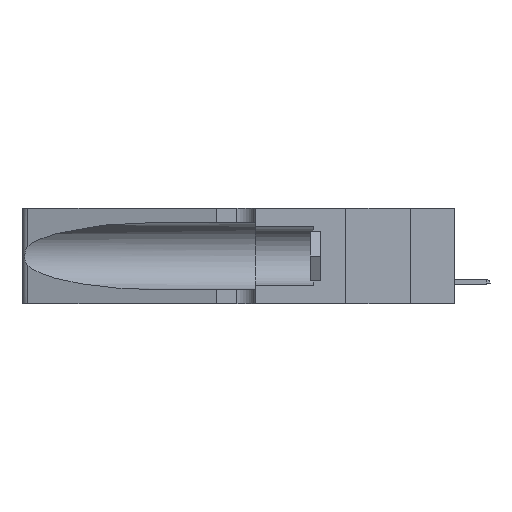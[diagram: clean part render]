
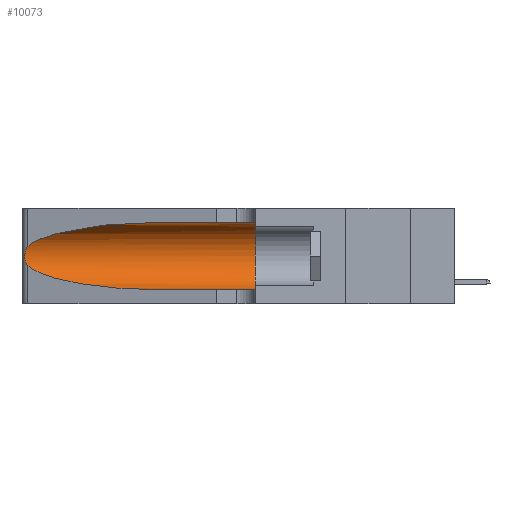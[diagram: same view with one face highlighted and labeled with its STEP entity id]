
A CAD part, left-side view. The second image highlights one B-rep face of the part: STEP entity #10073.
In plain terms, the highlighted cylindrical face has radius 3.308 mm (diameter 6.617 mm), a partial arc.
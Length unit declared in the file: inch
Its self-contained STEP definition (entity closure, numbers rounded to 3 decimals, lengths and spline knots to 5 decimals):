
#525 = DIRECTION ( 'NONE',  ( 0., -1., 0. ) ) ;
#949 = DIRECTION ( 'NONE',  ( 0., 0., -1. ) ) ;
#981 = CARTESIAN_POINT ( 'NONE',  ( 0.26075, 1.23896, 0.178 ) ) ;
#2021 = CARTESIAN_POINT ( 'NONE',  ( 0.18966, 0.96281, 0.31525 ) ) ;
#2221 = AXIS2_PLACEMENT_3D ( 'NONE', #19820, #525, #949 ) ;
#2693 = EDGE_CURVE ( 'NONE', #4115, #14118, #26232, .T. ) ;
#2950 = CARTESIAN_POINT ( 'NONE',  ( 0.25639, 1.23184, 0.21858 ) ) ;
#4115 = VERTEX_POINT ( 'NONE', #12184 ) ;
#4227 = EDGE_CURVE ( 'NONE', #4115, #12556, #16961, .T. ) ;
#4262 = CARTESIAN_POINT ( 'NONE',  ( 0.25487, 1.22718, 0.22369 ) ) ;
#4934 = CARTESIAN_POINT ( 'NONE',  ( 0.25555, 1.22993, 0.14849 ) ) ;
#5211 = CARTESIAN_POINT ( 'NONE',  ( 0.26017, 1.23833, 0.17102 ) ) ;
#5354 = CARTESIAN_POINT ( 'NONE',  ( 0.26075, 1.23896, 0.19203 ) ) ;
#6523 = CARTESIAN_POINT ( 'NONE',  ( 0.2373, 1.15595, 0.28018 ) ) ;
#6920 = CARTESIAN_POINT ( 'NONE',  ( 0.1305, 0.35, 0.05475 ) ) ;
#7315 = ORIENTED_EDGE ( 'NONE', *, *, #9658, .T. ) ;
#8468 = CARTESIAN_POINT ( 'NONE',  ( 0.2373, 1.15595, 0.08982 ) ) ;
#8658 = CARTESIAN_POINT ( 'NONE',  ( 0.1305, 0.72297, 0.31525 ) ) ;
#8821 = DIRECTION ( 'NONE',  ( 0., 0., 1. ) ) ;
#9414 = VERTEX_POINT ( 'NONE', #6920 ) ;
#9658 = EDGE_CURVE ( 'NONE', #12556, #23799, #11583, .T. ) ;
#9897 = CARTESIAN_POINT ( 'NONE',  ( 0.25487, 1.22718, 0.14631 ) ) ;
#10017 = CARTESIAN_POINT ( 'NONE',  ( 0.1305, 0.72297, 0.05475 ) ) ;
#10073 = ADVANCED_FACE ( 'NONE', ( #15599 ), #11262, .F. ) ;
#10475 =( BOUNDED_CURVE ( )  B_SPLINE_CURVE ( 3, ( #16762, #8468, #23089, #10017 ),
 .UNSPECIFIED., .F., .F. ) 
 B_SPLINE_CURVE_WITH_KNOTS ( ( 4, 4 ),
 ( 3.44316, 4.71239 ),
 .UNSPECIFIED. ) 
 CURVE ( )  GEOMETRIC_REPRESENTATION_ITEM ( )  RATIONAL_B_SPLINE_CURVE ( ( 1., 0.87, 0.87, 1. ) ) 
 REPRESENTATION_ITEM ( '' )  );
#10913 = EDGE_CURVE ( 'NONE', #23799, #18784, #10475, .T. ) ;
#11002 = LINE ( 'NONE', #19565, #17062 ) ;
#11262 = CYLINDRICAL_SURFACE ( 'NONE', #2221, 0.13025 ) ;
#11569 = CARTESIAN_POINT ( 'NONE',  ( 0.25487, 1.22718, 0.14631 ) ) ;
#11583 = B_SPLINE_CURVE_WITH_KNOTS ( 'NONE', 3,
 ( #22658, #16201, #2950, #24489, #17755, #15634, #5354, #981, #5211, #13813, #26738, #24213, #4934, #11569 ),
 .UNSPECIFIED., .F., .F.,
 ( 4, 2, 2, 2, 2, 2, 4 ),
 ( 0., 0.00027, 0.00053, 0.00107, 0.0016, 0.00187, 0.00214 ),
 .UNSPECIFIED. ) ;
#11917 = EDGE_CURVE ( 'NONE', #14118, #9414, #12728, .T. ) ;
#12184 = CARTESIAN_POINT ( 'NONE',  ( 0.1305, 0.72297, 0.31525 ) ) ;
#12556 = VERTEX_POINT ( 'NONE', #26222 ) ;
#12728 = CIRCLE ( 'NONE', #26154, 0.13025 ) ;
#13235 = EDGE_LOOP ( 'NONE', ( #14800, #7315, #13441, #21257, #23522, #22149 ) ) ;
#13441 = ORIENTED_EDGE ( 'NONE', *, *, #10913, .T. ) ;
#13813 = CARTESIAN_POINT ( 'NONE',  ( 0.25856, 1.23593, 0.16098 ) ) ;
#14118 = VERTEX_POINT ( 'NONE', #16528 ) ;
#14718 = DIRECTION ( 'NONE',  ( 0., 1., 0. ) ) ;
#14800 = ORIENTED_EDGE ( 'NONE', *, *, #4227, .T. ) ;
#15599 = FACE_OUTER_BOUND ( 'NONE', #13235, .T. ) ;
#15634 = CARTESIAN_POINT ( 'NONE',  ( 0.26018, 1.23835, 0.19895 ) ) ;
#16201 = CARTESIAN_POINT ( 'NONE',  ( 0.25555, 1.22994, 0.2215 ) ) ;
#16528 = CARTESIAN_POINT ( 'NONE',  ( 0.1305, 0.35, 0.31525 ) ) ;
#16762 = CARTESIAN_POINT ( 'NONE',  ( 0.25487, 1.22718, 0.14631 ) ) ;
#16961 =( BOUNDED_CURVE ( )  B_SPLINE_CURVE ( 3, ( #8658, #2021, #6523, #4262 ),
 .UNSPECIFIED., .F., .F. ) 
 B_SPLINE_CURVE_WITH_KNOTS ( ( 4, 4 ),
 ( 1.5708, 2.84003 ),
 .UNSPECIFIED. ) 
 CURVE ( )  GEOMETRIC_REPRESENTATION_ITEM ( )  RATIONAL_B_SPLINE_CURVE ( ( 1., 0.87, 0.87, 1. ) ) 
 REPRESENTATION_ITEM ( '' )  );
#17062 = VECTOR ( 'NONE', #17860, 39.37008 ) ;
#17755 = CARTESIAN_POINT ( 'NONE',  ( 0.25854, 1.2359, 0.20912 ) ) ;
#17860 = DIRECTION ( 'NONE',  ( 0., -1., 0. ) ) ;
#18081 = CARTESIAN_POINT ( 'NONE',  ( 0.1305, 1.61858, 0.31525 ) ) ;
#18221 = DIRECTION ( 'NONE',  ( 0., -1., 0. ) ) ;
#18784 = VERTEX_POINT ( 'NONE', #23599 ) ;
#19487 = CARTESIAN_POINT ( 'NONE',  ( 0.1305, 0.35, 0.185 ) ) ;
#19565 = CARTESIAN_POINT ( 'NONE',  ( 0.1305, 1.61858, 0.05475 ) ) ;
#19820 = CARTESIAN_POINT ( 'NONE',  ( 0.1305, 1.61858, 0.185 ) ) ;
#20377 = VECTOR ( 'NONE', #18221, 39.37008 ) ;
#20960 = EDGE_CURVE ( 'NONE', #18784, #9414, #11002, .T. ) ;
#21257 = ORIENTED_EDGE ( 'NONE', *, *, #20960, .T. ) ;
#22149 = ORIENTED_EDGE ( 'NONE', *, *, #2693, .F. ) ;
#22658 = CARTESIAN_POINT ( 'NONE',  ( 0.25487, 1.22718, 0.22369 ) ) ;
#23089 = CARTESIAN_POINT ( 'NONE',  ( 0.18966, 0.96281, 0.05475 ) ) ;
#23522 = ORIENTED_EDGE ( 'NONE', *, *, #11917, .F. ) ;
#23599 = CARTESIAN_POINT ( 'NONE',  ( 0.1305, 0.72297, 0.05475 ) ) ;
#23799 = VERTEX_POINT ( 'NONE', #9897 ) ;
#24213 = CARTESIAN_POINT ( 'NONE',  ( 0.25639, 1.23186, 0.15144 ) ) ;
#24489 = CARTESIAN_POINT ( 'NONE',  ( 0.25787, 1.23484, 0.2124 ) ) ;
#26154 = AXIS2_PLACEMENT_3D ( 'NONE', #19487, #14718, #8821 ) ;
#26222 = CARTESIAN_POINT ( 'NONE',  ( 0.25487, 1.22718, 0.22369 ) ) ;
#26232 = LINE ( 'NONE', #18081, #20377 ) ;
#26738 = CARTESIAN_POINT ( 'NONE',  ( 0.25789, 1.23486, 0.15765 ) ) ;
